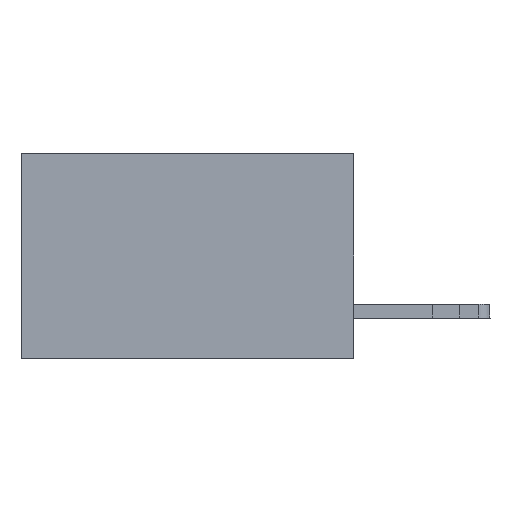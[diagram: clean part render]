
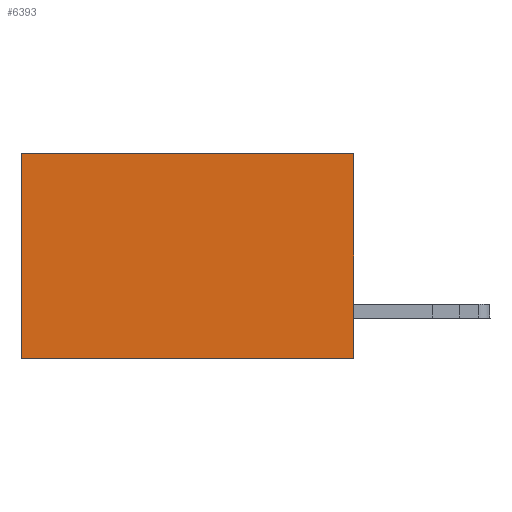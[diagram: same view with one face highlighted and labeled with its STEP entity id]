
A CAD part, left-side view. The second image highlights one B-rep face of the part: STEP entity #6393.
In plain terms, the highlighted planar face has unit normal (-1, 0, 0).
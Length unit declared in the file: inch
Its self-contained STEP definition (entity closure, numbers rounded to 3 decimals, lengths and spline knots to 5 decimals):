
#83 = EDGE_CURVE ( 'NONE', #13326, #22293, #22018, .T. ) ;
#575 = DIRECTION ( 'NONE',  ( 0., 1., 0. ) ) ;
#1184 = EDGE_LOOP ( 'NONE', ( #30021, #26634, #1742, #25322 ) ) ;
#1742 = ORIENTED_EDGE ( 'NONE', *, *, #24444, .F. ) ;
#3166 = CARTESIAN_POINT ( 'NONE',  ( 0.2875, 0., 0. ) ) ;
#3963 = FACE_OUTER_BOUND ( 'NONE', #1184, .T. ) ;
#4830 = CARTESIAN_POINT ( 'NONE',  ( 0.2875, 0., -0.37 ) ) ;
#5406 = LINE ( 'NONE', #8086, #29846 ) ;
#6393 = ADVANCED_FACE ( 'NONE', ( #3963 ), #7015, .F. ) ;
#6933 = CARTESIAN_POINT ( 'NONE',  ( 0.2875, 0.6, 0. ) ) ;
#7015 = PLANE ( 'NONE',  #9505 ) ;
#7102 = VERTEX_POINT ( 'NONE', #15314 ) ;
#8086 = CARTESIAN_POINT ( 'NONE',  ( 0.2875, 0., 0. ) ) ;
#8513 = CARTESIAN_POINT ( 'NONE',  ( 0.2875, 0., -0.37 ) ) ;
#8936 = DIRECTION ( 'NONE',  ( 0., 0., -1. ) ) ;
#9194 = CARTESIAN_POINT ( 'NONE',  ( 0.2875, 0.6, -0.37 ) ) ;
#9505 = AXIS2_PLACEMENT_3D ( 'NONE', #3166, #22644, #17825 ) ;
#11270 = VECTOR ( 'NONE', #16494, 39.37008 ) ;
#13151 = EDGE_CURVE ( 'NONE', #7102, #23659, #5406, .T. ) ;
#13326 = VERTEX_POINT ( 'NONE', #8513 ) ;
#14571 = DIRECTION ( 'NONE',  ( 0., 0., -1. ) ) ;
#15314 = CARTESIAN_POINT ( 'NONE',  ( 0.2875, 0., 0. ) ) ;
#16494 = DIRECTION ( 'NONE',  ( 0., 1., 0. ) ) ;
#17031 = CARTESIAN_POINT ( 'NONE',  ( 0.2875, 0.6, 0. ) ) ;
#17825 = DIRECTION ( 'NONE',  ( 0., 0., -1. ) ) ;
#18685 = LINE ( 'NONE', #23179, #22724 ) ;
#19542 = LINE ( 'NONE', #6933, #19979 ) ;
#19979 = VECTOR ( 'NONE', #14571, 39.37008 ) ;
#22018 = LINE ( 'NONE', #4830, #11270 ) ;
#22293 = VERTEX_POINT ( 'NONE', #9194 ) ;
#22644 = DIRECTION ( 'NONE',  ( 1., 0., 0. ) ) ;
#22724 = VECTOR ( 'NONE', #8936, 39.37008 ) ;
#23179 = CARTESIAN_POINT ( 'NONE',  ( 0.2875, 0., 0. ) ) ;
#23659 = VERTEX_POINT ( 'NONE', #17031 ) ;
#24444 = EDGE_CURVE ( 'NONE', #7102, #13326, #18685, .T. ) ;
#25322 = ORIENTED_EDGE ( 'NONE', *, *, #13151, .T. ) ;
#26634 = ORIENTED_EDGE ( 'NONE', *, *, #83, .F. ) ;
#29846 = VECTOR ( 'NONE', #575, 39.37008 ) ;
#30021 = ORIENTED_EDGE ( 'NONE', *, *, #30093, .T. ) ;
#30093 = EDGE_CURVE ( 'NONE', #23659, #22293, #19542, .T. ) ;
